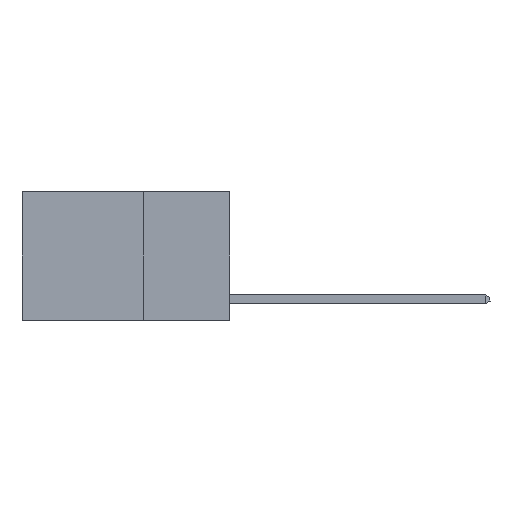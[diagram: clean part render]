
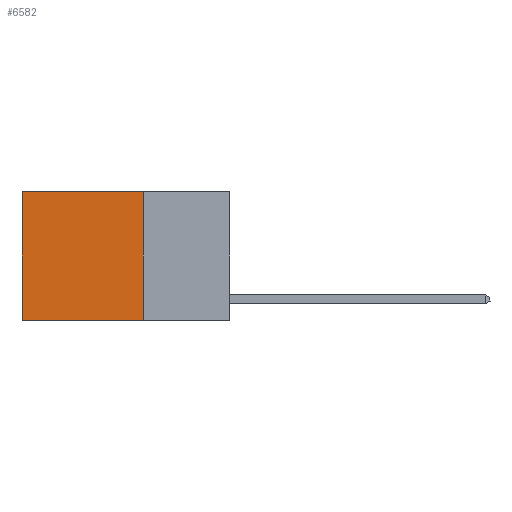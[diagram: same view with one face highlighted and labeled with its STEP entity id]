
A CAD part, left-side view. The second image highlights one B-rep face of the part: STEP entity #6582.
In plain terms, the highlighted planar face has unit normal (-1, 0, 0).
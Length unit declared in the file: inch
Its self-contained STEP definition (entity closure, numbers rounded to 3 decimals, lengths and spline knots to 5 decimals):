
#665 = VECTOR ( 'NONE', #14832, 39.37008 ) ;
#1311 = CARTESIAN_POINT ( 'NONE',  ( 0.2625, 0.25, -0.37 ) ) ;
#2888 = LINE ( 'NONE', #26875, #3547 ) ;
#3176 = CARTESIAN_POINT ( 'NONE',  ( 0.2625, 0.25, -0.37 ) ) ;
#3383 = CARTESIAN_POINT ( 'NONE',  ( 0.2625, 0.6, 0. ) ) ;
#3509 = ORIENTED_EDGE ( 'NONE', *, *, #25011, .F. ) ;
#3547 = VECTOR ( 'NONE', #24715, 39.37008 ) ;
#3549 = AXIS2_PLACEMENT_3D ( 'NONE', #10812, #25493, #12948 ) ;
#4695 = LINE ( 'NONE', #3176, #26658 ) ;
#5602 = LINE ( 'NONE', #3383, #26885 ) ;
#6582 = ADVANCED_FACE ( 'NONE', ( #19699 ), #25775, .F. ) ;
#7280 = CARTESIAN_POINT ( 'NONE',  ( 0.2625, 0.25, 0. ) ) ;
#7327 = ORIENTED_EDGE ( 'NONE', *, *, #20820, .T. ) ;
#7494 = VERTEX_POINT ( 'NONE', #1311 ) ;
#9367 = EDGE_LOOP ( 'NONE', ( #17778, #10548, #3509, #7327 ) ) ;
#10548 = ORIENTED_EDGE ( 'NONE', *, *, #19906, .F. ) ;
#10812 = CARTESIAN_POINT ( 'NONE',  ( 0.2625, 0.25, 0. ) ) ;
#12948 = DIRECTION ( 'NONE',  ( 0., 0., -1. ) ) ;
#13418 = CARTESIAN_POINT ( 'NONE',  ( 0.2625, 0.6, 0. ) ) ;
#14832 = DIRECTION ( 'NONE',  ( 0., 1., 0. ) ) ;
#15068 = CARTESIAN_POINT ( 'NONE',  ( 0.2625, 0.6, -0.37 ) ) ;
#15305 = EDGE_CURVE ( 'NONE', #19027, #19642, #5602, .T. ) ;
#16576 = LINE ( 'NONE', #16784, #665 ) ;
#16784 = CARTESIAN_POINT ( 'NONE',  ( 0.2625, 0.25, 0. ) ) ;
#17778 = ORIENTED_EDGE ( 'NONE', *, *, #15305, .T. ) ;
#17975 = DIRECTION ( 'NONE',  ( 0., 0., -1. ) ) ;
#19027 = VERTEX_POINT ( 'NONE', #13418 ) ;
#19642 = VERTEX_POINT ( 'NONE', #15068 ) ;
#19699 = FACE_OUTER_BOUND ( 'NONE', #9367, .T. ) ;
#19836 = VERTEX_POINT ( 'NONE', #7280 ) ;
#19906 = EDGE_CURVE ( 'NONE', #7494, #19642, #4695, .T. ) ;
#20438 = DIRECTION ( 'NONE',  ( 0., 1., 0. ) ) ;
#20820 = EDGE_CURVE ( 'NONE', #19836, #19027, #16576, .T. ) ;
#24715 = DIRECTION ( 'NONE',  ( 0., 0., -1. ) ) ;
#25011 = EDGE_CURVE ( 'NONE', #19836, #7494, #2888, .T. ) ;
#25493 = DIRECTION ( 'NONE',  ( 1., 0., 0. ) ) ;
#25775 = PLANE ( 'NONE',  #3549 ) ;
#26658 = VECTOR ( 'NONE', #20438, 39.37008 ) ;
#26875 = CARTESIAN_POINT ( 'NONE',  ( 0.2625, 0.25, 0. ) ) ;
#26885 = VECTOR ( 'NONE', #17975, 39.37008 ) ;
